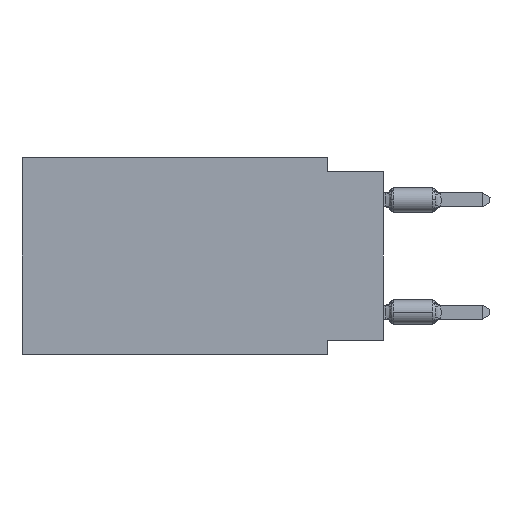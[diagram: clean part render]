
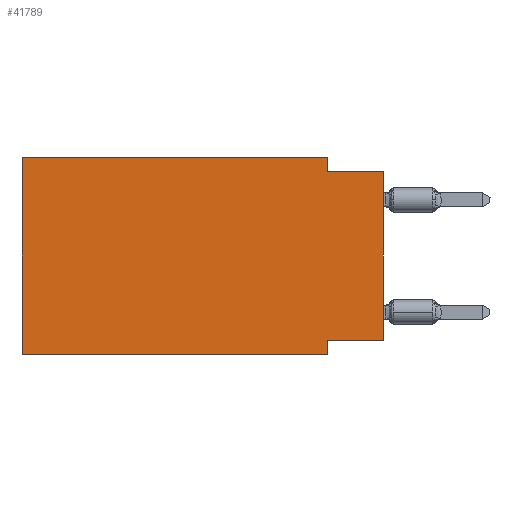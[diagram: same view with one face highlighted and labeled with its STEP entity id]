
A CAD part, left-side view. The second image highlights one B-rep face of the part: STEP entity #41789.
In plain terms, the highlighted planar face has unit normal (-1, 0, 0).
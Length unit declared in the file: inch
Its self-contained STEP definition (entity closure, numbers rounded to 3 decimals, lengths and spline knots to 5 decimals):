
#272 = ORIENTED_EDGE ( 'NONE', *, *, #19119, .F. ) ;
#1506 = ORIENTED_EDGE ( 'NONE', *, *, #10594, .F. ) ;
#1550 = VECTOR ( 'NONE', #10550, 39.37008 ) ;
#2093 = VERTEX_POINT ( 'NONE', #14991 ) ;
#2121 = LINE ( 'NONE', #18027, #5230 ) ;
#2278 = DIRECTION ( 'NONE',  ( 0., -1., 0. ) ) ;
#2300 = ORIENTED_EDGE ( 'NONE', *, *, #38689, .F. ) ;
#2420 = DIRECTION ( 'NONE',  ( 0., 0., 1. ) ) ;
#3897 = CARTESIAN_POINT ( 'NONE',  ( 0., 0.645, 0. ) ) ;
#5230 = VECTOR ( 'NONE', #14111, 39.37008 ) ;
#5308 = VERTEX_POINT ( 'NONE', #5579 ) ;
#5579 = CARTESIAN_POINT ( 'NONE',  ( 0., 0.1, -0.325 ) ) ;
#6153 = ORIENTED_EDGE ( 'NONE', *, *, #10555, .F. ) ;
#6211 = LINE ( 'NONE', #22137, #27511 ) ;
#6234 = ORIENTED_EDGE ( 'NONE', *, *, #18479, .F. ) ;
#7386 = DIRECTION ( 'NONE',  ( 0., 0., -1. ) ) ;
#7921 = LINE ( 'NONE', #38940, #48200 ) ;
#7983 = CARTESIAN_POINT ( 'NONE',  ( 0., 0.645, 0. ) ) ;
#8002 = EDGE_CURVE ( 'NONE', #49621, #35514, #35534, .T. ) ;
#10180 = VECTOR ( 'NONE', #2420, 39.37008 ) ;
#10550 = DIRECTION ( 'NONE',  ( 0., 1., 0. ) ) ;
#10555 = EDGE_CURVE ( 'NONE', #32567, #5308, #13713, .T. ) ;
#10594 = EDGE_CURVE ( 'NONE', #2093, #46540, #7921, .T. ) ;
#11384 = LINE ( 'NONE', #7983, #50286 ) ;
#13394 = CARTESIAN_POINT ( 'NONE',  ( 0., 0.1, -0.35 ) ) ;
#13713 = LINE ( 'NONE', #17865, #1550 ) ;
#14111 = DIRECTION ( 'NONE',  ( 0., 0., 1. ) ) ;
#14700 = LINE ( 'NONE', #18611, #10180 ) ;
#14991 = CARTESIAN_POINT ( 'NONE',  ( 0., 0.1, 0. ) ) ;
#16227 = CARTESIAN_POINT ( 'NONE',  ( 0., 0.645, -0.35 ) ) ;
#17865 = CARTESIAN_POINT ( 'NONE',  ( 0., 0., -0.325 ) ) ;
#18027 = CARTESIAN_POINT ( 'NONE',  ( 0., 0.645, 0. ) ) ;
#18479 = EDGE_CURVE ( 'NONE', #48696, #2093, #11384, .T. ) ;
#18611 = CARTESIAN_POINT ( 'NONE',  ( 0., 0., 0. ) ) ;
#18734 = CARTESIAN_POINT ( 'NONE',  ( 0., 0.1, -0.025 ) ) ;
#19119 = EDGE_CURVE ( 'NONE', #5308, #35514, #38120, .T. ) ;
#20094 = AXIS2_PLACEMENT_3D ( 'NONE', #25095, #44391, #40474 ) ;
#21063 = EDGE_LOOP ( 'NONE', ( #34464, #31514, #1506, #6234, #2300, #30250, #272, #6153 ) ) ;
#21508 = VECTOR ( 'NONE', #37884, 39.37008 ) ;
#22137 = CARTESIAN_POINT ( 'NONE',  ( 0., 0., -0.025 ) ) ;
#25095 = CARTESIAN_POINT ( 'NONE',  ( 0., 0.645, 0. ) ) ;
#27511 = VECTOR ( 'NONE', #2278, 39.37008 ) ;
#27722 = DIRECTION ( 'NONE',  ( 0., -1., 0. ) ) ;
#30250 = ORIENTED_EDGE ( 'NONE', *, *, #8002, .T. ) ;
#31374 = CARTESIAN_POINT ( 'NONE',  ( 0., 0.645, -0.35 ) ) ;
#31514 = ORIENTED_EDGE ( 'NONE', *, *, #47756, .F. ) ;
#32135 = FACE_OUTER_BOUND ( 'NONE', #21063, .T. ) ;
#32325 = CARTESIAN_POINT ( 'NONE',  ( 0., 0.1, -0.35 ) ) ;
#32567 = VERTEX_POINT ( 'NONE', #46015 ) ;
#34464 = ORIENTED_EDGE ( 'NONE', *, *, #38322, .T. ) ;
#35514 = VERTEX_POINT ( 'NONE', #32325 ) ;
#35534 = LINE ( 'NONE', #31374, #38947 ) ;
#37884 = DIRECTION ( 'NONE',  ( 0., 0., -1. ) ) ;
#38120 = LINE ( 'NONE', #13394, #21508 ) ;
#38322 = EDGE_CURVE ( 'NONE', #32567, #48459, #14700, .T. ) ;
#38689 = EDGE_CURVE ( 'NONE', #49621, #48696, #2121, .T. ) ;
#38940 = CARTESIAN_POINT ( 'NONE',  ( 0., 0.1, 0. ) ) ;
#38947 = VECTOR ( 'NONE', #27722, 39.37008 ) ;
#40474 = DIRECTION ( 'NONE',  ( 0., 0., -1. ) ) ;
#40991 = PLANE ( 'NONE',  #20094 ) ;
#41789 = ADVANCED_FACE ( 'NONE', ( #32135 ), #40991, .F. ) ;
#43177 = DIRECTION ( 'NONE',  ( 0., -1., 0. ) ) ;
#44391 = DIRECTION ( 'NONE',  ( 1., 0., 0. ) ) ;
#46015 = CARTESIAN_POINT ( 'NONE',  ( 0., 0., -0.325 ) ) ;
#46540 = VERTEX_POINT ( 'NONE', #18734 ) ;
#47756 = EDGE_CURVE ( 'NONE', #46540, #48459, #6211, .T. ) ;
#48200 = VECTOR ( 'NONE', #7386, 39.37008 ) ;
#48459 = VERTEX_POINT ( 'NONE', #48818 ) ;
#48696 = VERTEX_POINT ( 'NONE', #3897 ) ;
#48818 = CARTESIAN_POINT ( 'NONE',  ( 0., 0., -0.025 ) ) ;
#49621 = VERTEX_POINT ( 'NONE', #16227 ) ;
#50286 = VECTOR ( 'NONE', #43177, 39.37008 ) ;
